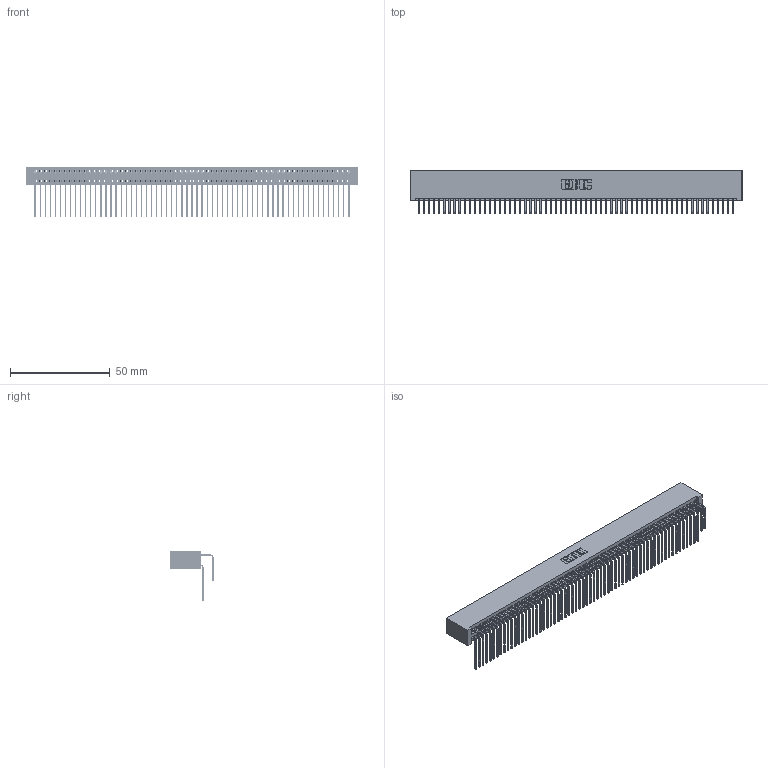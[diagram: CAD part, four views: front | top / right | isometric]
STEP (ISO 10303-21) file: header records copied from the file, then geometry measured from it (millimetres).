
FILE_DESCRIPTION (( 'STEP AP203' ), '1' );
FILE_NAME ('395-126-558-201.STEP', '2018-12-04T07:33:10', ( '' ), ( '' ), 'SwSTEP 2.0', 'SolidWorks 2016', '' );
FILE_SCHEMA (( 'CONFIG_CONTROL_DESIGN' ));
Length unit declared in the file: inch
Products named in the file (4): 345 Part_No Mounting Lugs; 345-292-001_558 559 Tail - 1; 345-292-001_558 Tail - 2; 395-126-558-201
Assembly tree (127 placements, depth 2):
  395-126-558-201
    345 Part_No Mounting Lugs
    345-292-001_558 559 Tail - 1  x63
    345-292-001_558 Tail - 2  x63
Bounding box: 166.62 x 21.83 x 25.53 mm (x, y, z)
Volume: 17723.7 mm3; surface area: 30326.6 mm2
Topology: 127 solids, 127 shells, 6670 faces, 19847 edges, 13062 vertices
Faces by surface type: plane 4486, cylinder 2184
Entity records: 47979 total; most frequent: CARTESIAN_POINT 8067, ORIENTED_EDGE 7950, DIRECTION 7055, EDGE_CURVE 3975, VECTOR 3559, LINE 3559, VERTEX_POINT 2646, AXIS2_PLACEMENT_3D 1748
